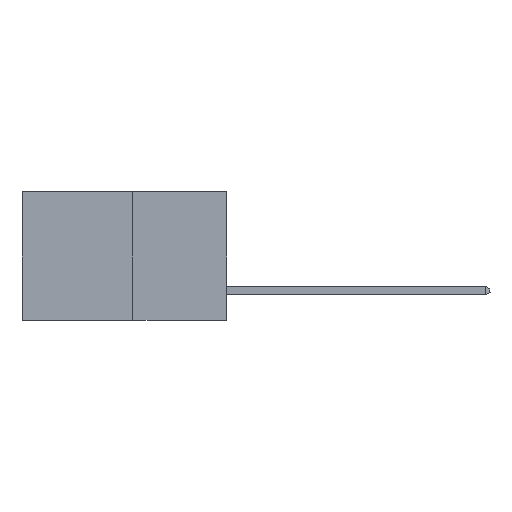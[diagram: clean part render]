
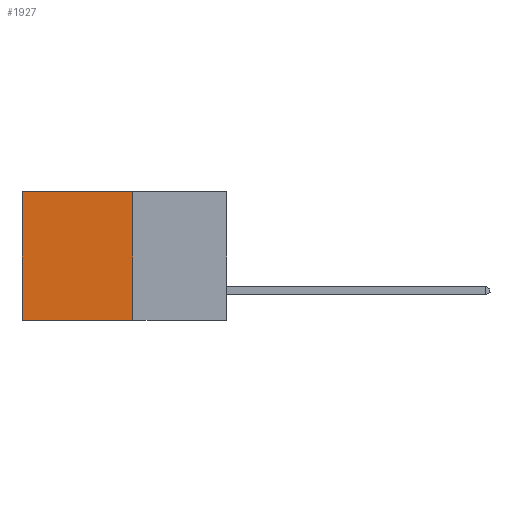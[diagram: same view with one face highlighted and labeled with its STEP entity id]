
A CAD part, left-side view. The second image highlights one B-rep face of the part: STEP entity #1927.
In plain terms, the highlighted planar face has unit normal (-1, 0, 0).
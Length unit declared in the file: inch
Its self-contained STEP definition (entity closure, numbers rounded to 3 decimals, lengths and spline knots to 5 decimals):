
#72 = VECTOR ( 'NONE', #627, 39.37008 ) ;
#627 = DIRECTION ( 'NONE',  ( 0., 0., -1. ) ) ;
#1103 = LINE ( 'NONE', #5128, #5644 ) ;
#1927 = ADVANCED_FACE ( 'NONE', ( #7849 ), #20984, .F. ) ;
#2143 = ORIENTED_EDGE ( 'NONE', *, *, #20024, .F. ) ;
#2506 = VERTEX_POINT ( 'NONE', #8461 ) ;
#2729 = EDGE_CURVE ( 'NONE', #14600, #2506, #17305, .T. ) ;
#4324 = DIRECTION ( 'NONE',  ( 0., 1., 0. ) ) ;
#4341 = CARTESIAN_POINT ( 'NONE',  ( 0.277, 0.27, 0. ) ) ;
#4381 = VECTOR ( 'NONE', #4324, 39.37008 ) ;
#4644 = LINE ( 'NONE', #7328, #72 ) ;
#5042 = DIRECTION ( 'NONE',  ( 0., 0., -1. ) ) ;
#5128 = CARTESIAN_POINT ( 'NONE',  ( 0.277, 0.27, -0.37 ) ) ;
#5644 = VECTOR ( 'NONE', #5042, 39.37008 ) ;
#5867 = EDGE_CURVE ( 'NONE', #14600, #8148, #1103, .T. ) ;
#6362 = DIRECTION ( 'NONE',  ( 0., 1., 0. ) ) ;
#7328 = CARTESIAN_POINT ( 'NONE',  ( 0.277, 0.59, -0.37 ) ) ;
#7849 = FACE_OUTER_BOUND ( 'NONE', #10722, .T. ) ;
#8148 = VERTEX_POINT ( 'NONE', #13219 ) ;
#8461 = CARTESIAN_POINT ( 'NONE',  ( 0.277, 0.59, 0. ) ) ;
#8625 = ORIENTED_EDGE ( 'NONE', *, *, #5867, .F. ) ;
#10250 = ORIENTED_EDGE ( 'NONE', *, *, #15217, .T. ) ;
#10722 = EDGE_LOOP ( 'NONE', ( #10250, #2143, #8625, #15378 ) ) ;
#10731 = VERTEX_POINT ( 'NONE', #11506 ) ;
#11506 = CARTESIAN_POINT ( 'NONE',  ( 0.277, 0.59, -0.37 ) ) ;
#12198 = LINE ( 'NONE', #21544, #21226 ) ;
#12965 = CARTESIAN_POINT ( 'NONE',  ( 0.277, 0.27, 0. ) ) ;
#13219 = CARTESIAN_POINT ( 'NONE',  ( 0.277, 0.27, -0.37 ) ) ;
#14600 = VERTEX_POINT ( 'NONE', #12965 ) ;
#15217 = EDGE_CURVE ( 'NONE', #2506, #10731, #4644, .T. ) ;
#15378 = ORIENTED_EDGE ( 'NONE', *, *, #2729, .T. ) ;
#17305 = LINE ( 'NONE', #4341, #4381 ) ;
#20024 = EDGE_CURVE ( 'NONE', #8148, #10731, #12198, .T. ) ;
#20189 = AXIS2_PLACEMENT_3D ( 'NONE', #21162, #20957, #20922 ) ;
#20922 = DIRECTION ( 'NONE',  ( 0., 0., -1. ) ) ;
#20957 = DIRECTION ( 'NONE',  ( 1., 0., 0. ) ) ;
#20984 = PLANE ( 'NONE',  #20189 ) ;
#21162 = CARTESIAN_POINT ( 'NONE',  ( 0.277, 0.27, -0.37 ) ) ;
#21226 = VECTOR ( 'NONE', #6362, 39.37008 ) ;
#21544 = CARTESIAN_POINT ( 'NONE',  ( 0.277, 0.27, -0.37 ) ) ;
